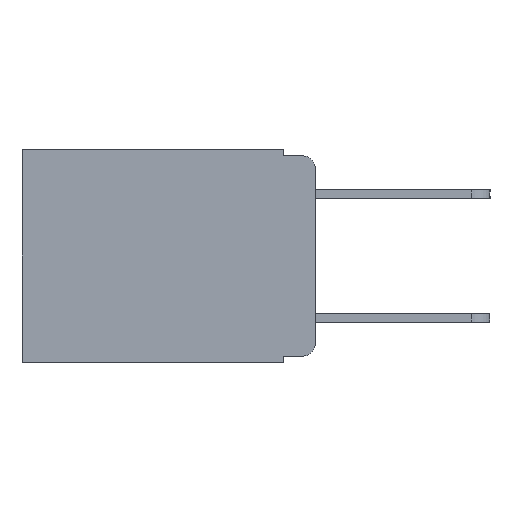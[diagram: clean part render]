
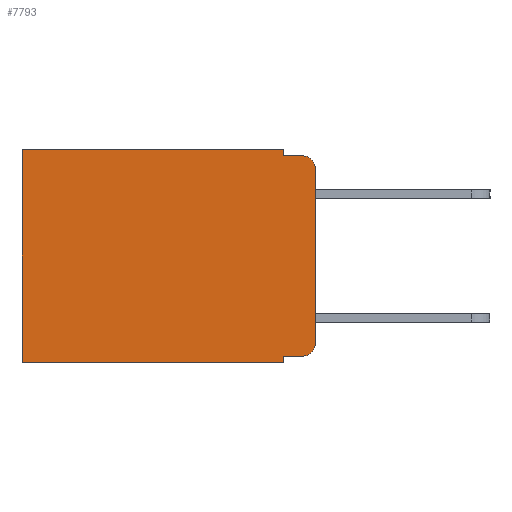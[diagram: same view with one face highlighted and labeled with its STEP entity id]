
A CAD part, left-side view. The second image highlights one B-rep face of the part: STEP entity #7793.
In plain terms, the highlighted planar face has unit normal (-1, 0, 0).
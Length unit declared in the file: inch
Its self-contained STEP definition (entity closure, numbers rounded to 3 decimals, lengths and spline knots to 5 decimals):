
#642 = EDGE_CURVE ( 'NONE', #4395, #2281, #10360, .T. ) ;
#711 = ORIENTED_EDGE ( 'NONE', *, *, #10669, .F. ) ;
#898 = DIRECTION ( 'NONE',  ( 1., 0., 0. ) ) ;
#934 = EDGE_CURVE ( 'NONE', #7335, #4902, #2102, .T. ) ;
#971 = ORIENTED_EDGE ( 'NONE', *, *, #10656, .T. ) ;
#1004 = CARTESIAN_POINT ( 'NONE',  ( 0.298, 0.051, 0. ) ) ;
#1020 = CARTESIAN_POINT ( 'NONE',  ( 0.298, 0., -0.03 ) ) ;
#1315 = ORIENTED_EDGE ( 'NONE', *, *, #4843, .F. ) ;
#1363 = ORIENTED_EDGE ( 'NONE', *, *, #10639, .F. ) ;
#1523 = ORIENTED_EDGE ( 'NONE', *, *, #934, .T. ) ;
#1585 = DIRECTION ( 'NONE',  ( 0., 1., 0. ) ) ;
#1640 = ORIENTED_EDGE ( 'NONE', *, *, #10673, .T. ) ;
#1741 = ORIENTED_EDGE ( 'NONE', *, *, #642, .F. ) ;
#1933 = AXIS2_PLACEMENT_3D ( 'NONE', #5237, #898, #5484 ) ;
#2099 = CARTESIAN_POINT ( 'NONE',  ( 0.298, 0., 0. ) ) ;
#2102 = LINE ( 'NONE', #8011, #6633 ) ;
#2154 = ORIENTED_EDGE ( 'NONE', *, *, #10716, .F. ) ;
#2281 = VERTEX_POINT ( 'NONE', #11183 ) ;
#2438 = DIRECTION ( 'NONE',  ( 0., -1., 0. ) ) ;
#2710 = ORIENTED_EDGE ( 'NONE', *, *, #10819, .T. ) ;
#2927 = LINE ( 'NONE', #4931, #7298 ) ;
#2997 = ORIENTED_EDGE ( 'NONE', *, *, #10884, .T. ) ;
#3134 = CARTESIAN_POINT ( 'NONE',  ( 0.298, 0.473, 0. ) ) ;
#3173 = DIRECTION ( 'NONE',  ( 0., 0., -1. ) ) ;
#3326 = CARTESIAN_POINT ( 'NONE',  ( 0.298, 0.051, 0. ) ) ;
#3562 = VECTOR ( 'NONE', #5686, 39.37008 ) ;
#3682 = CARTESIAN_POINT ( 'NONE',  ( 0.298, 0.02, -0.01 ) ) ;
#3937 = CIRCLE ( 'NONE', #4876, 0.02 ) ;
#3947 = VECTOR ( 'NONE', #1585, 39.37008 ) ;
#4006 = DIRECTION ( 'NONE',  ( -1., 0., 0. ) ) ;
#4120 = EDGE_LOOP ( 'NONE', ( #711, #971, #1315, #1363, #1523, #1640, #1741, #2154, #2710, #2997 ) ) ;
#4236 = CARTESIAN_POINT ( 'NONE',  ( 0.298, 0.02, -0.313 ) ) ;
#4395 = VERTEX_POINT ( 'NONE', #8656 ) ;
#4488 = VECTOR ( 'NONE', #5879, 39.37008 ) ;
#4830 = CARTESIAN_POINT ( 'NONE',  ( 0.298, 0.051, -0.01 ) ) ;
#4843 = EDGE_CURVE ( 'NONE', #6475, #6714, #5137, .T. ) ;
#4876 = AXIS2_PLACEMENT_3D ( 'NONE', #4236, #10091, #5129 ) ;
#4902 = VERTEX_POINT ( 'NONE', #3134 ) ;
#4931 = CARTESIAN_POINT ( 'NONE',  ( 0.298, 0.473, 0. ) ) ;
#5055 = LINE ( 'NONE', #1004, #7046 ) ;
#5129 = DIRECTION ( 'NONE',  ( 0., 0., -1. ) ) ;
#5137 = LINE ( 'NONE', #4830, #9356 ) ;
#5237 = CARTESIAN_POINT ( 'NONE',  ( 0.298, 0., 0. ) ) ;
#5484 = DIRECTION ( 'NONE',  ( 0., 0., -1. ) ) ;
#5571 = CIRCLE ( 'NONE', #8500, 0.02 ) ;
#5686 = DIRECTION ( 'NONE',  ( 0., 0., -1. ) ) ;
#5815 = DIRECTION ( 'NONE',  ( 0., 0., -1. ) ) ;
#5861 = LINE ( 'NONE', #9831, #3562 ) ;
#5879 = DIRECTION ( 'NONE',  ( 0., -1., 0. ) ) ;
#6083 = CARTESIAN_POINT ( 'NONE',  ( 0.298, 0.051, -0.333 ) ) ;
#6475 = VERTEX_POINT ( 'NONE', #8733 ) ;
#6633 = VECTOR ( 'NONE', #8024, 39.37008 ) ;
#6686 = FACE_OUTER_BOUND ( 'NONE', #4120, .T. ) ;
#6714 = VERTEX_POINT ( 'NONE', #3682 ) ;
#7046 = VECTOR ( 'NONE', #3173, 39.37008 ) ;
#7158 = CARTESIAN_POINT ( 'NONE',  ( 0.298, 0., -0.313 ) ) ;
#7298 = VECTOR ( 'NONE', #5815, 39.37008 ) ;
#7335 = VERTEX_POINT ( 'NONE', #3326 ) ;
#7450 = DIRECTION ( 'NONE',  ( 0., 0., -1. ) ) ;
#7544 = LINE ( 'NONE', #2099, #9986 ) ;
#7547 = CARTESIAN_POINT ( 'NONE',  ( 0.298, 0.051, -0.333 ) ) ;
#7739 = VERTEX_POINT ( 'NONE', #6083 ) ;
#7793 = ADVANCED_FACE ( 'NONE', ( #6686 ), #10913, .F. ) ;
#8011 = CARTESIAN_POINT ( 'NONE',  ( 0.298, 0., 0. ) ) ;
#8024 = DIRECTION ( 'NONE',  ( 0., 1., 0. ) ) ;
#8500 = AXIS2_PLACEMENT_3D ( 'NONE', #9128, #4006, #9893 ) ;
#8632 = VERTEX_POINT ( 'NONE', #9647 ) ;
#8656 = CARTESIAN_POINT ( 'NONE',  ( 0.298, 0.051, -0.343 ) ) ;
#8733 = CARTESIAN_POINT ( 'NONE',  ( 0.298, 0.051, -0.01 ) ) ;
#8908 = CARTESIAN_POINT ( 'NONE',  ( 0.298, 0., -0.343 ) ) ;
#9128 = CARTESIAN_POINT ( 'NONE',  ( 0.298, 0.02, -0.03 ) ) ;
#9356 = VECTOR ( 'NONE', #2438, 39.37008 ) ;
#9516 = VERTEX_POINT ( 'NONE', #7158 ) ;
#9647 = CARTESIAN_POINT ( 'NONE',  ( 0.298, 0.02, -0.333 ) ) ;
#9808 = VERTEX_POINT ( 'NONE', #1020 ) ;
#9831 = CARTESIAN_POINT ( 'NONE',  ( 0.298, 0.051, 0. ) ) ;
#9893 = DIRECTION ( 'NONE',  ( 0., 0., -1. ) ) ;
#9986 = VECTOR ( 'NONE', #7450, 39.37008 ) ;
#10091 = DIRECTION ( 'NONE',  ( -1., 0., 0. ) ) ;
#10360 = LINE ( 'NONE', #8908, #3947 ) ;
#10639 = EDGE_CURVE ( 'NONE', #7335, #6475, #5861, .T. ) ;
#10656 = EDGE_CURVE ( 'NONE', #9808, #6714, #5571, .T. ) ;
#10669 = EDGE_CURVE ( 'NONE', #9808, #9516, #7544, .T. ) ;
#10673 = EDGE_CURVE ( 'NONE', #4902, #2281, #2927, .T. ) ;
#10716 = EDGE_CURVE ( 'NONE', #7739, #4395, #5055, .T. ) ;
#10813 = LINE ( 'NONE', #7547, #4488 ) ;
#10819 = EDGE_CURVE ( 'NONE', #7739, #8632, #10813, .T. ) ;
#10884 = EDGE_CURVE ( 'NONE', #8632, #9516, #3937, .T. ) ;
#10913 = PLANE ( 'NONE',  #1933 ) ;
#11183 = CARTESIAN_POINT ( 'NONE',  ( 0.298, 0.473, -0.343 ) ) ;
